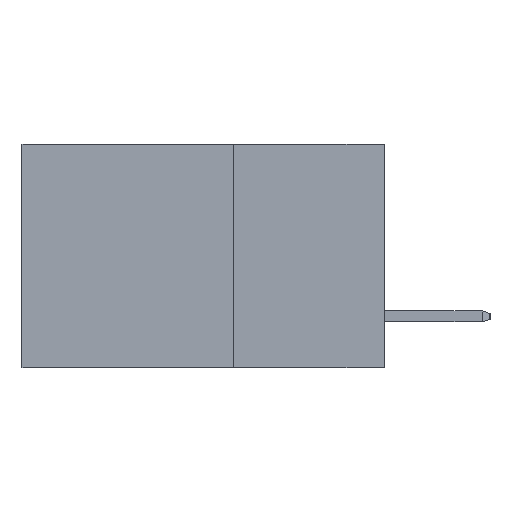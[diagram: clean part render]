
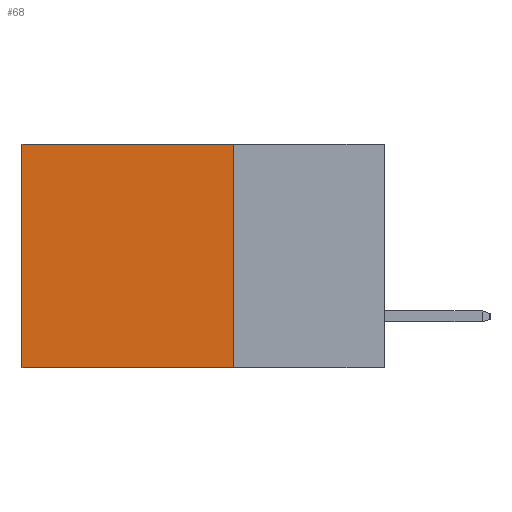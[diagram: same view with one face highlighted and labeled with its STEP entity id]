
A CAD part, left-side view. The second image highlights one B-rep face of the part: STEP entity #68.
In plain terms, the highlighted planar face has unit normal (-1, 0, 0).
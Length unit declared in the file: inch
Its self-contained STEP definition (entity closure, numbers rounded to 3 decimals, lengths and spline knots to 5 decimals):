
#68 = ADVANCED_FACE ( 'NONE', ( #14220 ), #14960, .F. ) ;
#229 = DIRECTION ( 'NONE',  ( 0., 1., 0. ) ) ;
#1146 = CARTESIAN_POINT ( 'NONE',  ( 0.298, 0.25, 0. ) ) ;
#2113 = CARTESIAN_POINT ( 'NONE',  ( 0.298, 0.25, -0.37 ) ) ;
#2181 = VERTEX_POINT ( 'NONE', #10655 ) ;
#2361 = LINE ( 'NONE', #2113, #5778 ) ;
#2378 = CARTESIAN_POINT ( 'NONE',  ( 0.298, 0.6, -0.37 ) ) ;
#4141 = LINE ( 'NONE', #16946, #14580 ) ;
#5616 = VERTEX_POINT ( 'NONE', #10003 ) ;
#5688 = ORIENTED_EDGE ( 'NONE', *, *, #14600, .T. ) ;
#5778 = VECTOR ( 'NONE', #13538, 39.37008 ) ;
#5827 = VERTEX_POINT ( 'NONE', #2378 ) ;
#5959 = LINE ( 'NONE', #1146, #9311 ) ;
#6223 = LINE ( 'NONE', #8934, #9566 ) ;
#7621 = AXIS2_PLACEMENT_3D ( 'NONE', #15648, #14386, #14344 ) ;
#7846 = EDGE_CURVE ( 'NONE', #2181, #5616, #5959, .T. ) ;
#7958 = EDGE_CURVE ( 'NONE', #8772, #5827, #4141, .T. ) ;
#8487 = ORIENTED_EDGE ( 'NONE', *, *, #15272, .F. ) ;
#8772 = VERTEX_POINT ( 'NONE', #14616 ) ;
#8934 = CARTESIAN_POINT ( 'NONE',  ( 0.298, 0.25, 0. ) ) ;
#9311 = VECTOR ( 'NONE', #15445, 39.37008 ) ;
#9566 = VECTOR ( 'NONE', #229, 39.37008 ) ;
#10003 = CARTESIAN_POINT ( 'NONE',  ( 0.298, 0.25, -0.37 ) ) ;
#10655 = CARTESIAN_POINT ( 'NONE',  ( 0.298, 0.25, 0. ) ) ;
#13538 = DIRECTION ( 'NONE',  ( 0., 1., 0. ) ) ;
#14220 = FACE_OUTER_BOUND ( 'NONE', #15527, .T. ) ;
#14344 = DIRECTION ( 'NONE',  ( 0., 0., -1. ) ) ;
#14386 = DIRECTION ( 'NONE',  ( 1., 0., 0. ) ) ;
#14580 = VECTOR ( 'NONE', #18377, 39.37008 ) ;
#14600 = EDGE_CURVE ( 'NONE', #2181, #8772, #6223, .T. ) ;
#14616 = CARTESIAN_POINT ( 'NONE',  ( 0.298, 0.6, 0. ) ) ;
#14960 = PLANE ( 'NONE',  #7621 ) ;
#15272 = EDGE_CURVE ( 'NONE', #5616, #5827, #2361, .T. ) ;
#15445 = DIRECTION ( 'NONE',  ( 0., 0., -1. ) ) ;
#15527 = EDGE_LOOP ( 'NONE', ( #18199, #8487, #15971, #5688 ) ) ;
#15648 = CARTESIAN_POINT ( 'NONE',  ( 0.298, 0.25, 0. ) ) ;
#15971 = ORIENTED_EDGE ( 'NONE', *, *, #7846, .F. ) ;
#16946 = CARTESIAN_POINT ( 'NONE',  ( 0.298, 0.6, 0. ) ) ;
#18199 = ORIENTED_EDGE ( 'NONE', *, *, #7958, .T. ) ;
#18377 = DIRECTION ( 'NONE',  ( 0., 0., -1. ) ) ;
